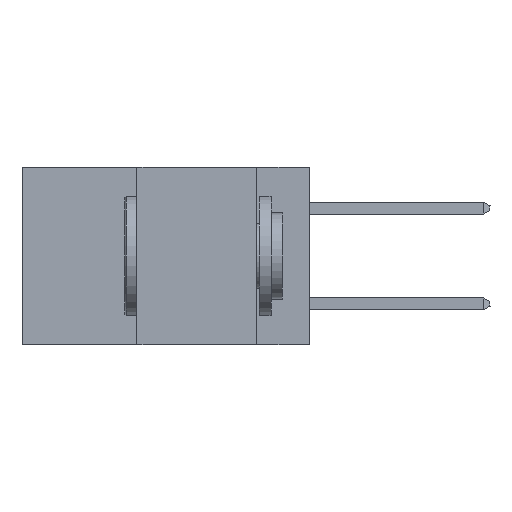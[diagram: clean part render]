
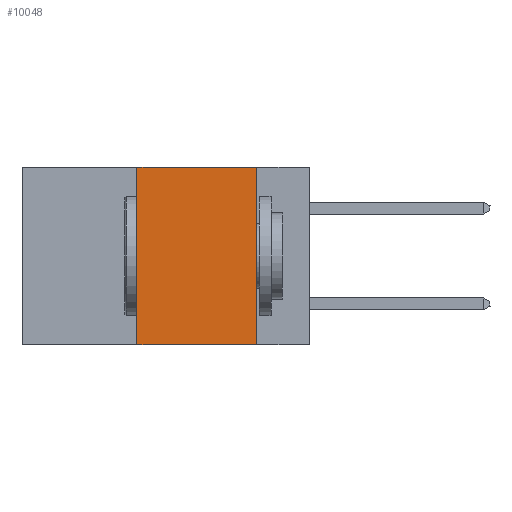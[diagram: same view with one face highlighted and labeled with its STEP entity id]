
A CAD part, left-side view. The second image highlights one B-rep face of the part: STEP entity #10048.
In plain terms, the highlighted planar face has unit normal (-1, 0, 0).
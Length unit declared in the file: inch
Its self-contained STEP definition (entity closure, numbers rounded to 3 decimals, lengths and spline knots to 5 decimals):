
#1435 = DIRECTION ( 'NONE',  ( 0., -1., 0. ) ) ;
#1769 = DIRECTION ( 'NONE',  ( 0., 0., -1. ) ) ;
#1921 = FACE_OUTER_BOUND ( 'NONE', #13046, .T. ) ;
#2090 = VECTOR ( 'NONE', #6794, 39.37008 ) ;
#3261 = VERTEX_POINT ( 'NONE', #20718 ) ;
#4965 = VECTOR ( 'NONE', #19634, 39.37008 ) ;
#6137 = VERTEX_POINT ( 'NONE', #22584 ) ;
#6437 = LINE ( 'NONE', #19873, #4965 ) ;
#6794 = DIRECTION ( 'NONE',  ( 0., -1., 0. ) ) ;
#6820 = VERTEX_POINT ( 'NONE', #23659 ) ;
#7057 = LINE ( 'NONE', #15872, #2090 ) ;
#7069 = CARTESIAN_POINT ( 'NONE',  ( 0., 0.6, 0. ) ) ;
#7627 = CARTESIAN_POINT ( 'NONE',  ( 0., 0.6, 0. ) ) ;
#9344 = DIRECTION ( 'NONE',  ( 1., 0., 0. ) ) ;
#9909 = VERTEX_POINT ( 'NONE', #15127 ) ;
#10048 = ADVANCED_FACE ( 'NONE', ( #1921 ), #16564, .F. ) ;
#10534 = DIRECTION ( 'NONE',  ( 0., 0., 1. ) ) ;
#13046 = EDGE_LOOP ( 'NONE', ( #17409, #19247, #15012, #18314 ) ) ;
#14038 = LINE ( 'NONE', #7069, #16641 ) ;
#15012 = ORIENTED_EDGE ( 'NONE', *, *, #22423, .F. ) ;
#15127 = CARTESIAN_POINT ( 'NONE',  ( 0., 0.36, -0.37 ) ) ;
#15519 = LINE ( 'NONE', #20380, #20470 ) ;
#15872 = CARTESIAN_POINT ( 'NONE',  ( 0., 0.6, -0.37 ) ) ;
#16564 = PLANE ( 'NONE',  #20629 ) ;
#16641 = VECTOR ( 'NONE', #1435, 39.37008 ) ;
#16698 = EDGE_CURVE ( 'NONE', #6820, #6137, #14038, .T. ) ;
#17149 = EDGE_CURVE ( 'NONE', #6137, #3261, #6437, .T. ) ;
#17409 = ORIENTED_EDGE ( 'NONE', *, *, #17149, .F. ) ;
#18314 = ORIENTED_EDGE ( 'NONE', *, *, #23602, .T. ) ;
#19247 = ORIENTED_EDGE ( 'NONE', *, *, #16698, .F. ) ;
#19634 = DIRECTION ( 'NONE',  ( 0., 0., -1. ) ) ;
#19873 = CARTESIAN_POINT ( 'NONE',  ( 0., 0.11, 0. ) ) ;
#20380 = CARTESIAN_POINT ( 'NONE',  ( 0., 0.36, 0. ) ) ;
#20470 = VECTOR ( 'NONE', #10534, 39.37008 ) ;
#20629 = AXIS2_PLACEMENT_3D ( 'NONE', #7627, #9344, #1769 ) ;
#20718 = CARTESIAN_POINT ( 'NONE',  ( 0., 0.11, -0.37 ) ) ;
#22423 = EDGE_CURVE ( 'NONE', #9909, #6820, #15519, .T. ) ;
#22584 = CARTESIAN_POINT ( 'NONE',  ( 0., 0.11, 0. ) ) ;
#23602 = EDGE_CURVE ( 'NONE', #9909, #3261, #7057, .T. ) ;
#23659 = CARTESIAN_POINT ( 'NONE',  ( 0., 0.36, 0. ) ) ;
